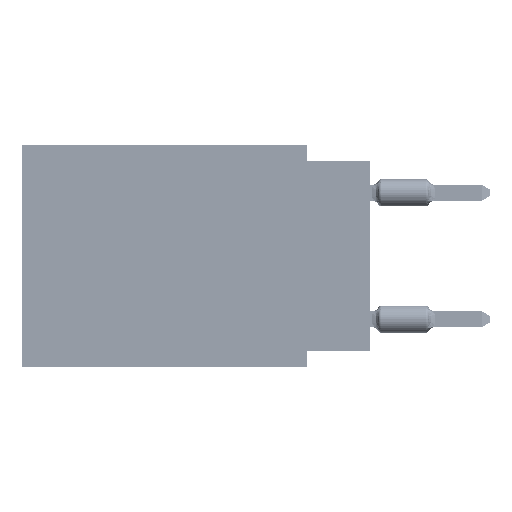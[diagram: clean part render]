
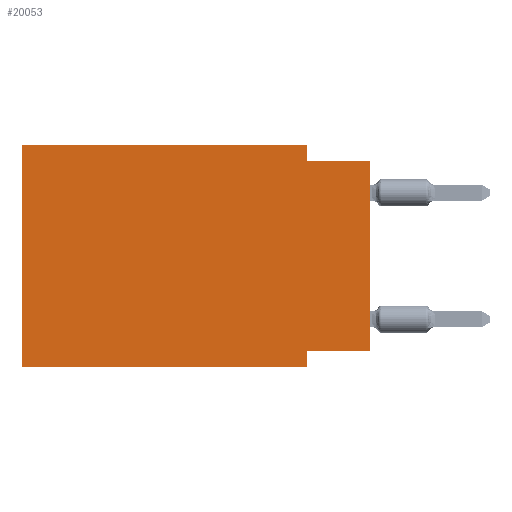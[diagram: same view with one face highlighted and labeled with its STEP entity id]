
A CAD part, left-side view. The second image highlights one B-rep face of the part: STEP entity #20053.
In plain terms, the highlighted planar face has unit normal (-1, 0, 0).
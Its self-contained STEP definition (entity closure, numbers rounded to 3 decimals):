
#554 = VECTOR ( 'NONE', #77032, 1000. ) ;
#851 = EDGE_CURVE ( 'NONE', #20403, #9016, #89343, .T. ) ;
#2367 = DIRECTION ( 'NONE',  ( 0., -1., 0. ) ) ;
#4992 = EDGE_CURVE ( 'NONE', #9016, #13787, #16219, .T. ) ;
#6101 = AXIS2_PLACEMENT_3D ( 'NONE', #68138, #38674, #61242 ) ;
#6874 = VECTOR ( 'NONE', #89798, 1000. ) ;
#8396 = DIRECTION ( 'NONE',  ( 0., 1., 0. ) ) ;
#9016 = VERTEX_POINT ( 'NONE', #10187 ) ;
#9264 = ORIENTED_EDGE ( 'NONE', *, *, #81464, .F. ) ;
#9721 = LINE ( 'NONE', #23956, #66273 ) ;
#10187 = CARTESIAN_POINT ( 'NONE',  ( 0., 2.54, -8.255 ) ) ;
#11066 = VERTEX_POINT ( 'NONE', #88995 ) ;
#12707 = CARTESIAN_POINT ( 'NONE',  ( 0., 2.54, 0. ) ) ;
#13787 = VERTEX_POINT ( 'NONE', #51089 ) ;
#15175 = EDGE_CURVE ( 'NONE', #34659, #96732, #54955, .T. ) ;
#15843 = VECTOR ( 'NONE', #56700, 1000. ) ;
#16219 = LINE ( 'NONE', #31399, #554 ) ;
#20053 = ADVANCED_FACE ( 'NONE', ( #31805 ), #38199, .F. ) ;
#20403 = VERTEX_POINT ( 'NONE', #50858 ) ;
#22925 = ORIENTED_EDGE ( 'NONE', *, *, #45536, .F. ) ;
#23956 = CARTESIAN_POINT ( 'NONE',  ( 0., 13.97, -8.89 ) ) ;
#24413 = LINE ( 'NONE', #59375, #6874 ) ;
#25031 = CARTESIAN_POINT ( 'NONE',  ( 0., 0., -0.635 ) ) ;
#26332 = CARTESIAN_POINT ( 'NONE',  ( 0., 0., -0.635 ) ) ;
#26374 = EDGE_CURVE ( 'NONE', #20403, #96732, #30326, .T. ) ;
#26710 = LINE ( 'NONE', #27695, #40034 ) ;
#27695 = CARTESIAN_POINT ( 'NONE',  ( 0., 13.97, 0. ) ) ;
#29906 = ORIENTED_EDGE ( 'NONE', *, *, #26374, .T. ) ;
#30326 = LINE ( 'NONE', #60252, #69850 ) ;
#31399 = CARTESIAN_POINT ( 'NONE',  ( 0., 2.54, -8.89 ) ) ;
#31805 = FACE_OUTER_BOUND ( 'NONE', #73586, .T. ) ;
#34659 = VERTEX_POINT ( 'NONE', #50741 ) ;
#38199 = PLANE ( 'NONE',  #6101 ) ;
#38674 = DIRECTION ( 'NONE',  ( 1., 0., 0. ) ) ;
#40034 = VECTOR ( 'NONE', #48792, 1000. ) ;
#41516 = VERTEX_POINT ( 'NONE', #12707 ) ;
#45536 = EDGE_CURVE ( 'NONE', #41516, #34659, #24413, .T. ) ;
#45811 = VERTEX_POINT ( 'NONE', #96919 ) ;
#48354 = CARTESIAN_POINT ( 'NONE',  ( 0., 13.97, 0. ) ) ;
#48792 = DIRECTION ( 'NONE',  ( 0., -1., 0. ) ) ;
#48812 = VECTOR ( 'NONE', #8396, 1000. ) ;
#50741 = CARTESIAN_POINT ( 'NONE',  ( 0., 2.54, -0.635 ) ) ;
#50858 = CARTESIAN_POINT ( 'NONE',  ( 0., 0., -8.255 ) ) ;
#51089 = CARTESIAN_POINT ( 'NONE',  ( 0., 2.54, -8.89 ) ) ;
#52621 = EDGE_CURVE ( 'NONE', #45811, #13787, #9721, .T. ) ;
#54955 = LINE ( 'NONE', #25031, #74046 ) ;
#55730 = LINE ( 'NONE', #48354, #15843 ) ;
#56700 = DIRECTION ( 'NONE',  ( 0., 0., 1. ) ) ;
#59375 = CARTESIAN_POINT ( 'NONE',  ( 0., 2.54, 0. ) ) ;
#60252 = CARTESIAN_POINT ( 'NONE',  ( 0., 0., 0. ) ) ;
#61242 = DIRECTION ( 'NONE',  ( 0., 0., -1. ) ) ;
#66273 = VECTOR ( 'NONE', #2367, 1000. ) ;
#66612 = ORIENTED_EDGE ( 'NONE', *, *, #4992, .F. ) ;
#67268 = CARTESIAN_POINT ( 'NONE',  ( 0., 0., -8.255 ) ) ;
#68138 = CARTESIAN_POINT ( 'NONE',  ( 0., 13.97, 0. ) ) ;
#69433 = ORIENTED_EDGE ( 'NONE', *, *, #851, .F. ) ;
#69850 = VECTOR ( 'NONE', #73036, 1000. ) ;
#71576 = EDGE_CURVE ( 'NONE', #11066, #41516, #26710, .T. ) ;
#71618 = ORIENTED_EDGE ( 'NONE', *, *, #15175, .F. ) ;
#73036 = DIRECTION ( 'NONE',  ( 0., 0., 1. ) ) ;
#73586 = EDGE_LOOP ( 'NONE', ( #29906, #71618, #22925, #81853, #9264, #79883, #66612, #69433 ) ) ;
#74046 = VECTOR ( 'NONE', #77539, 1000. ) ;
#77032 = DIRECTION ( 'NONE',  ( 0., 0., -1. ) ) ;
#77539 = DIRECTION ( 'NONE',  ( 0., -1., 0. ) ) ;
#79883 = ORIENTED_EDGE ( 'NONE', *, *, #52621, .T. ) ;
#81464 = EDGE_CURVE ( 'NONE', #45811, #11066, #55730, .T. ) ;
#81853 = ORIENTED_EDGE ( 'NONE', *, *, #71576, .F. ) ;
#88995 = CARTESIAN_POINT ( 'NONE',  ( 0., 13.97, 0. ) ) ;
#89343 = LINE ( 'NONE', #67268, #48812 ) ;
#89798 = DIRECTION ( 'NONE',  ( 0., 0., -1. ) ) ;
#96732 = VERTEX_POINT ( 'NONE', #26332 ) ;
#96919 = CARTESIAN_POINT ( 'NONE',  ( 0., 13.97, -8.89 ) ) ;
